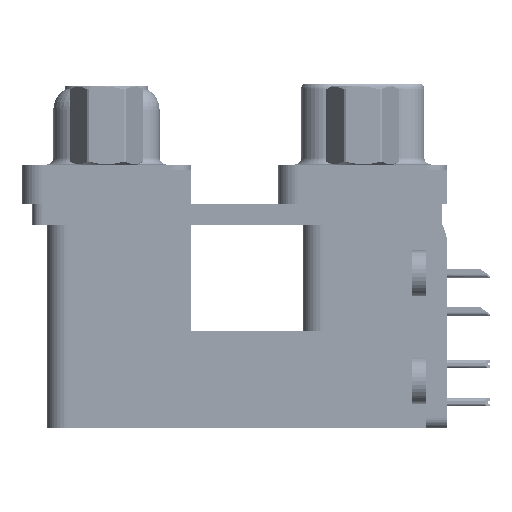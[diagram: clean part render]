
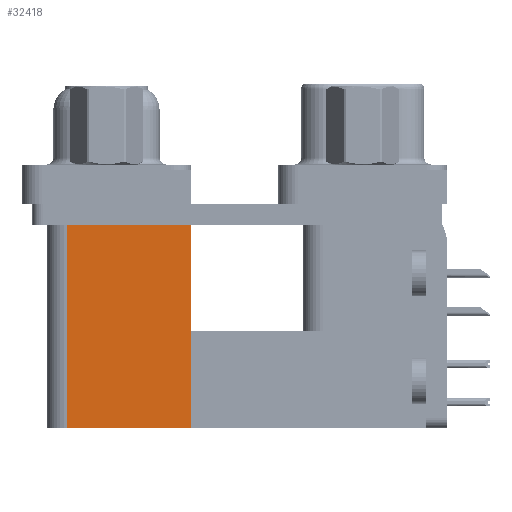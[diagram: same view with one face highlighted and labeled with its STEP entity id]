
A CAD part, left-side view. The second image highlights one B-rep face of the part: STEP entity #32418.
In plain terms, the highlighted planar face has unit normal (-1, 0, 0).
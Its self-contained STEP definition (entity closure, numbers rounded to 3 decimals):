
#8 = CARTESIAN_POINT ( 'NONE',  ( 3.7, 21.975, -19.2 ) ) ;
#3487 = CARTESIAN_POINT ( 'NONE',  ( 3.7, 12.775, -19.2 ) ) ;
#6094 = VERTEX_POINT ( 'NONE', #38811 ) ;
#7717 = VECTOR ( 'NONE', #26187, 1000. ) ;
#10614 = CARTESIAN_POINT ( 'NONE',  ( 3.7, 12.775, -19.2 ) ) ;
#11915 = DIRECTION ( 'NONE',  ( 0., 1., 0. ) ) ;
#12537 = LINE ( 'NONE', #60028, #33383 ) ;
#13574 = VERTEX_POINT ( 'NONE', #43430 ) ;
#14576 = EDGE_CURVE ( 'NONE', #44908, #13574, #20187, .T. ) ;
#16448 = LINE ( 'NONE', #26496, #7717 ) ;
#20067 = EDGE_CURVE ( 'NONE', #6094, #13574, #16448, .T. ) ;
#20187 = LINE ( 'NONE', #39399, #61646 ) ;
#20371 = CARTESIAN_POINT ( 'NONE',  ( 3.7, 12.775, -19.2 ) ) ;
#20991 = DIRECTION ( 'NONE',  ( 1., 0., 0. ) ) ;
#22272 = VECTOR ( 'NONE', #53707, 1000. ) ;
#25106 = FACE_OUTER_BOUND ( 'NONE', #50358, .T. ) ;
#26187 = DIRECTION ( 'NONE',  ( 0., 1., 0. ) ) ;
#26496 = CARTESIAN_POINT ( 'NONE',  ( 3.7, 12.775, -2.5 ) ) ;
#29632 = ORIENTED_EDGE ( 'NONE', *, *, #20067, .T. ) ;
#32418 = ADVANCED_FACE ( 'NONE', ( #25106 ), #44321, .F. ) ;
#33383 = VECTOR ( 'NONE', #11915, 1000. ) ;
#34855 = DIRECTION ( 'NONE',  ( 0., 0., -1. ) ) ;
#35439 = LINE ( 'NONE', #10614, #22272 ) ;
#37627 = ORIENTED_EDGE ( 'NONE', *, *, #46040, .T. ) ;
#38811 = CARTESIAN_POINT ( 'NONE',  ( 3.7, 12.775, -2.5 ) ) ;
#39399 = CARTESIAN_POINT ( 'NONE',  ( 3.7, 21.975, -19.2 ) ) ;
#39704 = DIRECTION ( 'NONE',  ( 0., 0., 1. ) ) ;
#43430 = CARTESIAN_POINT ( 'NONE',  ( 3.7, 21.975, -2.5 ) ) ;
#44321 = PLANE ( 'NONE',  #44910 ) ;
#44908 = VERTEX_POINT ( 'NONE', #8 ) ;
#44910 = AXIS2_PLACEMENT_3D ( 'NONE', #20371, #20991, #34855 ) ;
#46040 = EDGE_CURVE ( 'NONE', #54134, #6094, #35439, .T. ) ;
#46345 = ORIENTED_EDGE ( 'NONE', *, *, #46563, .F. ) ;
#46563 = EDGE_CURVE ( 'NONE', #54134, #44908, #12537, .T. ) ;
#50358 = EDGE_LOOP ( 'NONE', ( #29632, #58377, #46345, #37627 ) ) ;
#53707 = DIRECTION ( 'NONE',  ( 0., 0., 1. ) ) ;
#54134 = VERTEX_POINT ( 'NONE', #3487 ) ;
#58377 = ORIENTED_EDGE ( 'NONE', *, *, #14576, .F. ) ;
#60028 = CARTESIAN_POINT ( 'NONE',  ( 3.7, 12.775, -19.2 ) ) ;
#61646 = VECTOR ( 'NONE', #39704, 1000. ) ;
